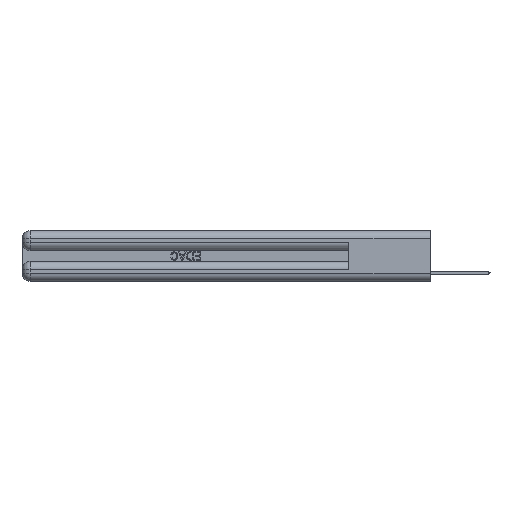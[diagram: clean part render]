
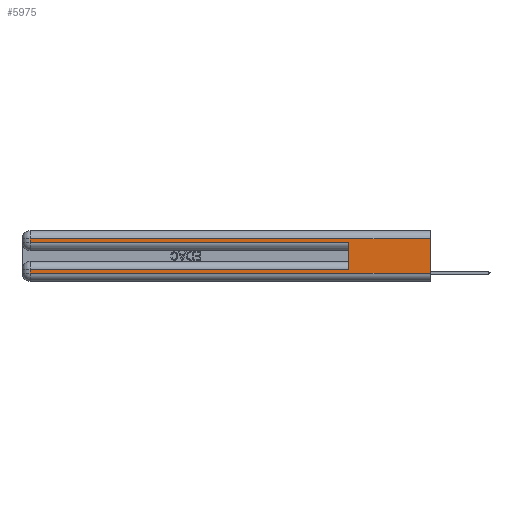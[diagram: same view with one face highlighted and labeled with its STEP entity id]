
A CAD part, left-side view. The second image highlights one B-rep face of the part: STEP entity #5975.
In plain terms, the highlighted planar face has unit normal (-1, 0, 0).
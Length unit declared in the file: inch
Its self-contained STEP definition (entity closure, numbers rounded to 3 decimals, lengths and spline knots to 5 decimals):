
#7 = DIRECTION ( 'NONE',  ( 0., 0., 1. ) ) ;
#69 = CARTESIAN_POINT ( 'NONE',  ( 0., 0., 0.31 ) ) ;
#88 = DIRECTION ( 'NONE',  ( 1., 0., 0. ) ) ;
#775 = VECTOR ( 'NONE', #20387, 39.37008 ) ;
#838 = CARTESIAN_POINT ( 'NONE',  ( 0., 0., 0.37 ) ) ;
#1113 = EDGE_CURVE ( 'NONE', #15123, #20476, #1588, .T. ) ;
#1483 = LINE ( 'NONE', #69, #4668 ) ;
#1588 = LINE ( 'NONE', #19628, #27679 ) ;
#2536 = CARTESIAN_POINT ( 'NONE',  ( 0., 2.94, 0.37 ) ) ;
#3003 = DIRECTION ( 'NONE',  ( 0., 0., -1. ) ) ;
#4668 = VECTOR ( 'NONE', #10225, 39.37008 ) ;
#5898 = VERTEX_POINT ( 'NONE', #19590 ) ;
#5951 = VECTOR ( 'NONE', #29992, 39.37008 ) ;
#5975 = ADVANCED_FACE ( 'NONE', ( #9696 ), #22681, .F. ) ;
#6472 = ORIENTED_EDGE ( 'NONE', *, *, #21333, .F. ) ;
#6621 = LINE ( 'NONE', #25633, #25152 ) ;
#7210 = CARTESIAN_POINT ( 'NONE',  ( 0., 2.94, 0.285 ) ) ;
#7534 = VERTEX_POINT ( 'NONE', #27002 ) ;
#7732 = CARTESIAN_POINT ( 'NONE',  ( 0., 0.6, 0.085 ) ) ;
#7999 = VERTEX_POINT ( 'NONE', #24128 ) ;
#9696 = FACE_OUTER_BOUND ( 'NONE', #22027, .T. ) ;
#10029 = VERTEX_POINT ( 'NONE', #7210 ) ;
#10127 = DIRECTION ( 'NONE',  ( 0., 0., -1. ) ) ;
#10225 = DIRECTION ( 'NONE',  ( 0., 1., 0. ) ) ;
#10851 = VERTEX_POINT ( 'NONE', #12454 ) ;
#12454 = CARTESIAN_POINT ( 'NONE',  ( 0., 0.6, 0.285 ) ) ;
#13224 = VECTOR ( 'NONE', #23634, 39.37008 ) ;
#14543 = ORIENTED_EDGE ( 'NONE', *, *, #1113, .T. ) ;
#15031 = CARTESIAN_POINT ( 'NONE',  ( 0., 0., 0.06 ) ) ;
#15123 = VERTEX_POINT ( 'NONE', #7732 ) ;
#15578 = EDGE_CURVE ( 'NONE', #20476, #19382, #17333, .T. ) ;
#16079 = EDGE_CURVE ( 'NONE', #7534, #7999, #1483, .T. ) ;
#16240 = EDGE_CURVE ( 'NONE', #7534, #5898, #18445, .T. ) ;
#17203 = DIRECTION ( 'NONE',  ( 0., 1., 0. ) ) ;
#17333 = LINE ( 'NONE', #2536, #775 ) ;
#18153 = CARTESIAN_POINT ( 'NONE',  ( 0., 2.94, 0.085 ) ) ;
#18445 = LINE ( 'NONE', #838, #23566 ) ;
#19078 = EDGE_CURVE ( 'NONE', #7999, #10029, #6621, .T. ) ;
#19382 = VERTEX_POINT ( 'NONE', #31819 ) ;
#19590 = CARTESIAN_POINT ( 'NONE',  ( 0., 0., 0.06 ) ) ;
#19628 = CARTESIAN_POINT ( 'NONE',  ( 0., 0., 0.085 ) ) ;
#19835 = LINE ( 'NONE', #20381, #31762 ) ;
#20152 = CARTESIAN_POINT ( 'NONE',  ( 0., 0., 0.37 ) ) ;
#20381 = CARTESIAN_POINT ( 'NONE',  ( 0., 0.6, 0.145 ) ) ;
#20387 = DIRECTION ( 'NONE',  ( 0., 0., -1. ) ) ;
#20476 = VERTEX_POINT ( 'NONE', #18153 ) ;
#20616 = EDGE_CURVE ( 'NONE', #10029, #10851, #26640, .T. ) ;
#21333 = EDGE_CURVE ( 'NONE', #15123, #10851, #19835, .T. ) ;
#22027 = EDGE_LOOP ( 'NONE', ( #28199, #25073, #24808, #31093, #6472, #14543, #27220, #26804 ) ) ;
#22681 = PLANE ( 'NONE',  #26339 ) ;
#22896 = EDGE_CURVE ( 'NONE', #19382, #5898, #23314, .T. ) ;
#23314 = LINE ( 'NONE', #15031, #5951 ) ;
#23566 = VECTOR ( 'NONE', #31855, 39.37008 ) ;
#23634 = DIRECTION ( 'NONE',  ( 0., -1., 0. ) ) ;
#24128 = CARTESIAN_POINT ( 'NONE',  ( 0., 2.94, 0.31 ) ) ;
#24808 = ORIENTED_EDGE ( 'NONE', *, *, #19078, .T. ) ;
#25073 = ORIENTED_EDGE ( 'NONE', *, *, #16079, .T. ) ;
#25152 = VECTOR ( 'NONE', #3003, 39.37008 ) ;
#25633 = CARTESIAN_POINT ( 'NONE',  ( 0., 2.94, 0.37 ) ) ;
#26339 = AXIS2_PLACEMENT_3D ( 'NONE', #20152, #88, #10127 ) ;
#26640 = LINE ( 'NONE', #28524, #13224 ) ;
#26804 = ORIENTED_EDGE ( 'NONE', *, *, #22896, .T. ) ;
#27002 = CARTESIAN_POINT ( 'NONE',  ( 0., 0., 0.31 ) ) ;
#27220 = ORIENTED_EDGE ( 'NONE', *, *, #15578, .T. ) ;
#27679 = VECTOR ( 'NONE', #17203, 39.37008 ) ;
#28199 = ORIENTED_EDGE ( 'NONE', *, *, #16240, .F. ) ;
#28524 = CARTESIAN_POINT ( 'NONE',  ( 0., 0., 0.285 ) ) ;
#29992 = DIRECTION ( 'NONE',  ( 0., -1., 0. ) ) ;
#31093 = ORIENTED_EDGE ( 'NONE', *, *, #20616, .T. ) ;
#31762 = VECTOR ( 'NONE', #7, 39.37008 ) ;
#31819 = CARTESIAN_POINT ( 'NONE',  ( 0., 2.94, 0.06 ) ) ;
#31855 = DIRECTION ( 'NONE',  ( 0., 0., -1. ) ) ;
